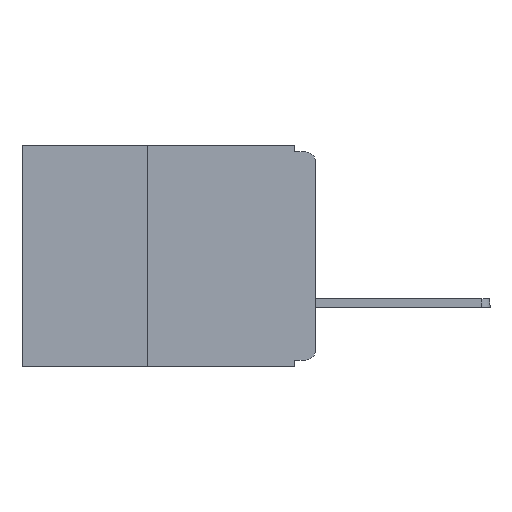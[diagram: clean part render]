
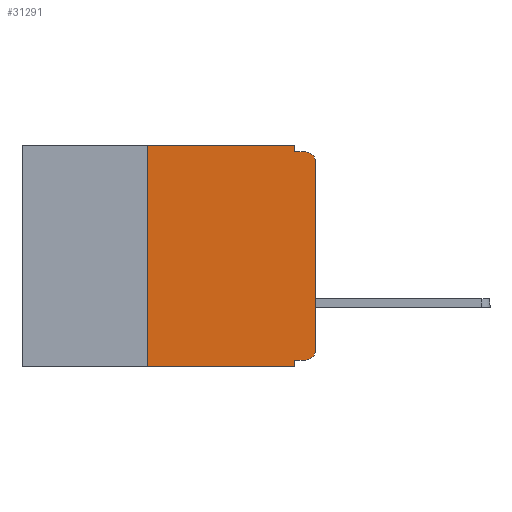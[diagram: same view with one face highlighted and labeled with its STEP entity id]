
A CAD part, left-side view. The second image highlights one B-rep face of the part: STEP entity #31291.
In plain terms, the highlighted planar face has unit normal (-1, 0, 0).
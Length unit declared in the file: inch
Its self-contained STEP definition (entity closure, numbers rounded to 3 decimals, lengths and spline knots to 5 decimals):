
#246 = EDGE_CURVE ( 'NONE', #33086, #11292, #21087, .T. ) ;
#701 = AXIS2_PLACEMENT_3D ( 'NONE', #18425, #2061, #21121 ) ;
#761 = VECTOR ( 'NONE', #15464, 39.37008 ) ;
#796 = ORIENTED_EDGE ( 'NONE', *, *, #28040, .F. ) ;
#2061 = DIRECTION ( 'NONE',  ( -1., 0., 0. ) ) ;
#2543 = VERTEX_POINT ( 'NONE', #17361 ) ;
#2847 = CARTESIAN_POINT ( 'NONE',  ( 0., 0.437, 0. ) ) ;
#3122 = VECTOR ( 'NONE', #30030, 39.37008 ) ;
#3256 = EDGE_CURVE ( 'NONE', #22504, #14102, #8245, .T. ) ;
#3585 = ORIENTED_EDGE ( 'NONE', *, *, #30733, .F. ) ;
#4159 = ORIENTED_EDGE ( 'NONE', *, *, #26108, .T. ) ;
#5030 = LINE ( 'NONE', #23716, #19453 ) ;
#5693 = DIRECTION ( 'NONE',  ( 0., 0., -1. ) ) ;
#5700 = PLANE ( 'NONE',  #23905 ) ;
#5894 = CARTESIAN_POINT ( 'NONE',  ( 0., 0., -0.01 ) ) ;
#6057 = EDGE_LOOP ( 'NONE', ( #17563, #28494, #8749, #3585, #20413, #28594, #26205, #796, #30922, #4159 ) ) ;
#7651 = DIRECTION ( 'NONE',  ( 0., 0., 1. ) ) ;
#7797 = VECTOR ( 'NONE', #8359, 39.37008 ) ;
#8245 = LINE ( 'NONE', #26086, #761 ) ;
#8359 = DIRECTION ( 'NONE',  ( 0., 1., 0. ) ) ;
#8491 = DIRECTION ( 'NONE',  ( 1., 0., 0. ) ) ;
#8523 = CARTESIAN_POINT ( 'NONE',  ( 0., 0.437, 0. ) ) ;
#8749 = ORIENTED_EDGE ( 'NONE', *, *, #10342, .F. ) ;
#8895 = AXIS2_PLACEMENT_3D ( 'NONE', #11176, #29868, #13895 ) ;
#10072 = CARTESIAN_POINT ( 'NONE',  ( 0., 0.031, -0.32 ) ) ;
#10288 = VECTOR ( 'NONE', #5693, 39.37008 ) ;
#10342 = EDGE_CURVE ( 'NONE', #2543, #11969, #18617, .T. ) ;
#11176 = CARTESIAN_POINT ( 'NONE',  ( 0., 0.015, -0.305 ) ) ;
#11218 = CIRCLE ( 'NONE', #8895, 0.015 ) ;
#11292 = VERTEX_POINT ( 'NONE', #11849 ) ;
#11849 = CARTESIAN_POINT ( 'NONE',  ( 0., 0.031, -0.33 ) ) ;
#11938 = CARTESIAN_POINT ( 'NONE',  ( 0., 0., -0.305 ) ) ;
#11948 = LINE ( 'NONE', #29875, #10288 ) ;
#11969 = VERTEX_POINT ( 'NONE', #22834 ) ;
#12549 = FACE_OUTER_BOUND ( 'NONE', #6057, .T. ) ;
#13641 = CARTESIAN_POINT ( 'NONE',  ( 0., 0.437, -0.33 ) ) ;
#13644 = CARTESIAN_POINT ( 'NONE',  ( 0., 0., -0.32 ) ) ;
#13895 = DIRECTION ( 'NONE',  ( 0., 0., -1. ) ) ;
#14090 = DIRECTION ( 'NONE',  ( 0., -1., 0. ) ) ;
#14102 = VERTEX_POINT ( 'NONE', #16316 ) ;
#15170 = EDGE_CURVE ( 'NONE', #33086, #26872, #5030, .T. ) ;
#15464 = DIRECTION ( 'NONE',  ( 0., 0., 1. ) ) ;
#16316 = CARTESIAN_POINT ( 'NONE',  ( 0., 0., -0.025 ) ) ;
#17361 = CARTESIAN_POINT ( 'NONE',  ( 0., 0.031, -0.01 ) ) ;
#17563 = ORIENTED_EDGE ( 'NONE', *, *, #3256, .T. ) ;
#18089 = CARTESIAN_POINT ( 'NONE',  ( 0., 0.031, 0. ) ) ;
#18175 = LINE ( 'NONE', #8523, #23601 ) ;
#18425 = CARTESIAN_POINT ( 'NONE',  ( 0., 0.015, -0.025 ) ) ;
#18617 = LINE ( 'NONE', #5894, #22362 ) ;
#19453 = VECTOR ( 'NONE', #7651, 39.37008 ) ;
#20413 = ORIENTED_EDGE ( 'NONE', *, *, #29311, .F. ) ;
#21087 = LINE ( 'NONE', #13641, #34336 ) ;
#21121 = DIRECTION ( 'NONE',  ( 0., 0., -1. ) ) ;
#21773 = DIRECTION ( 'NONE',  ( 0., -1., 0. ) ) ;
#22281 = VERTEX_POINT ( 'NONE', #24391 ) ;
#22362 = VECTOR ( 'NONE', #14090, 39.37008 ) ;
#22374 = CARTESIAN_POINT ( 'NONE',  ( 0., 0.25, 0. ) ) ;
#22504 = VERTEX_POINT ( 'NONE', #11938 ) ;
#22834 = CARTESIAN_POINT ( 'NONE',  ( 0., 0.015, -0.01 ) ) ;
#23601 = VECTOR ( 'NONE', #27237, 39.37008 ) ;
#23716 = CARTESIAN_POINT ( 'NONE',  ( 0., 0.25, -0.33 ) ) ;
#23905 = AXIS2_PLACEMENT_3D ( 'NONE', #2847, #8491, #27209 ) ;
#24391 = CARTESIAN_POINT ( 'NONE',  ( 0., 0.015, -0.32 ) ) ;
#24725 = VERTEX_POINT ( 'NONE', #18089 ) ;
#24743 = LINE ( 'NONE', #30143, #3122 ) ;
#26086 = CARTESIAN_POINT ( 'NONE',  ( 0., 0., 0. ) ) ;
#26108 = EDGE_CURVE ( 'NONE', #22281, #22504, #11218, .T. ) ;
#26205 = ORIENTED_EDGE ( 'NONE', *, *, #246, .T. ) ;
#26872 = VERTEX_POINT ( 'NONE', #22374 ) ;
#27209 = DIRECTION ( 'NONE',  ( 0., 0., -1. ) ) ;
#27237 = DIRECTION ( 'NONE',  ( 0., -1., 0. ) ) ;
#28040 = EDGE_CURVE ( 'NONE', #29042, #11292, #11948, .T. ) ;
#28297 = LINE ( 'NONE', #13644, #7797 ) ;
#28494 = ORIENTED_EDGE ( 'NONE', *, *, #33931, .T. ) ;
#28594 = ORIENTED_EDGE ( 'NONE', *, *, #15170, .F. ) ;
#29042 = VERTEX_POINT ( 'NONE', #10072 ) ;
#29311 = EDGE_CURVE ( 'NONE', #26872, #24725, #18175, .T. ) ;
#29412 = CARTESIAN_POINT ( 'NONE',  ( 0., 0.25, -0.33 ) ) ;
#29868 = DIRECTION ( 'NONE',  ( -1., 0., 0. ) ) ;
#29875 = CARTESIAN_POINT ( 'NONE',  ( 0., 0.031, -0.33 ) ) ;
#29941 = CIRCLE ( 'NONE', #701, 0.015 ) ;
#30030 = DIRECTION ( 'NONE',  ( 0., 0., -1. ) ) ;
#30143 = CARTESIAN_POINT ( 'NONE',  ( 0., 0.031, 0. ) ) ;
#30733 = EDGE_CURVE ( 'NONE', #24725, #2543, #24743, .T. ) ;
#30922 = ORIENTED_EDGE ( 'NONE', *, *, #33524, .F. ) ;
#31291 = ADVANCED_FACE ( 'NONE', ( #12549 ), #5700, .F. ) ;
#33086 = VERTEX_POINT ( 'NONE', #29412 ) ;
#33524 = EDGE_CURVE ( 'NONE', #22281, #29042, #28297, .T. ) ;
#33931 = EDGE_CURVE ( 'NONE', #14102, #11969, #29941, .T. ) ;
#34336 = VECTOR ( 'NONE', #21773, 39.37008 ) ;
